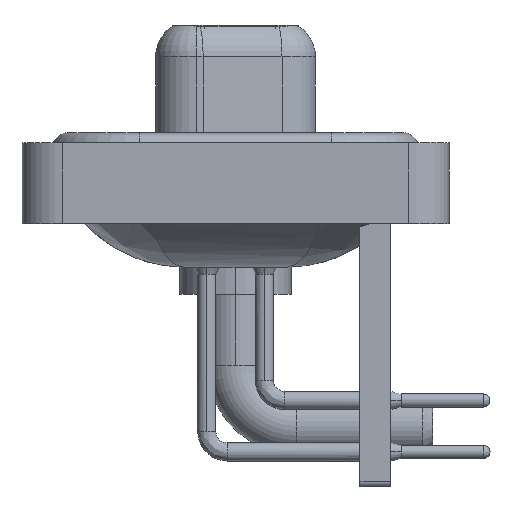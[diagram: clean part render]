
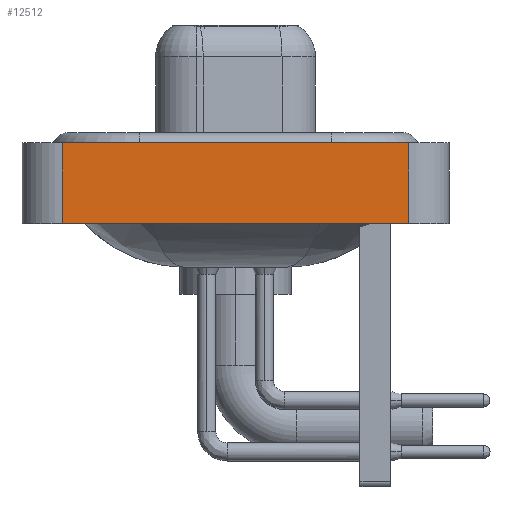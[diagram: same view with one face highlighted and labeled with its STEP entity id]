
A CAD part, left-side view. The second image highlights one B-rep face of the part: STEP entity #12512.
In plain terms, the highlighted planar face has unit normal (-1, 0, 0).
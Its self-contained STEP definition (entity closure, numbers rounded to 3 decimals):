
#1322 = FACE_OUTER_BOUND ( 'NONE', #2373, .T. ) ;
#1960 = DIRECTION ( 'NONE',  ( 0., 0., 1. ) ) ;
#2230 = DIRECTION ( 'NONE',  ( 0., 0., 1. ) ) ;
#2296 = LINE ( 'NONE', #13627, #19000 ) ;
#2373 = EDGE_LOOP ( 'NONE', ( #7023, #11223, #7813, #7846 ) ) ;
#2807 = LINE ( 'NONE', #15602, #14955 ) ;
#3771 = CARTESIAN_POINT ( 'NONE',  ( -7.25, -8.55, -3.6 ) ) ;
#3973 = EDGE_CURVE ( 'NONE', #20625, #4179, #2296, .T. ) ;
#4179 = VERTEX_POINT ( 'NONE', #20316 ) ;
#4591 = AXIS2_PLACEMENT_3D ( 'NONE', #19046, #11079, #2230 ) ;
#4674 = DIRECTION ( 'NONE',  ( 0., -1., 0. ) ) ;
#7023 = ORIENTED_EDGE ( 'NONE', *, *, #14893, .T. ) ;
#7077 = LINE ( 'NONE', #10123, #9894 ) ;
#7105 = DIRECTION ( 'NONE',  ( 0., -1., 0. ) ) ;
#7813 = ORIENTED_EDGE ( 'NONE', *, *, #8123, .F. ) ;
#7846 = ORIENTED_EDGE ( 'NONE', *, *, #8810, .T. ) ;
#8016 = VERTEX_POINT ( 'NONE', #3771 ) ;
#8123 = EDGE_CURVE ( 'NONE', #19703, #20625, #16268, .T. ) ;
#8810 = EDGE_CURVE ( 'NONE', #19703, #8016, #2807, .T. ) ;
#9894 = VECTOR ( 'NONE', #1960, 1000. ) ;
#10123 = CARTESIAN_POINT ( 'NONE',  ( -7.25, -8.55, -3.6 ) ) ;
#10589 = CARTESIAN_POINT ( 'NONE',  ( -7.25, 8.55, 0.4 ) ) ;
#11079 = DIRECTION ( 'NONE',  ( -1., 0., 0. ) ) ;
#11223 = ORIENTED_EDGE ( 'NONE', *, *, #3973, .F. ) ;
#11663 = DIRECTION ( 'NONE',  ( 0., 0., 1. ) ) ;
#11761 = CARTESIAN_POINT ( 'NONE',  ( -7.25, 8.55, -3.6 ) ) ;
#12512 = ADVANCED_FACE ( 'NONE', ( #1322 ), #20617, .T. ) ;
#13627 = CARTESIAN_POINT ( 'NONE',  ( -7.25, -8.55, 0.4 ) ) ;
#14893 = EDGE_CURVE ( 'NONE', #8016, #4179, #7077, .T. ) ;
#14955 = VECTOR ( 'NONE', #4674, 1000. ) ;
#15283 = VECTOR ( 'NONE', #11663, 1000. ) ;
#15602 = CARTESIAN_POINT ( 'NONE',  ( -7.25, -8.55, -3.6 ) ) ;
#16268 = LINE ( 'NONE', #11761, #15283 ) ;
#19000 = VECTOR ( 'NONE', #7105, 1000. ) ;
#19046 = CARTESIAN_POINT ( 'NONE',  ( -7.25, -8.55, -3.6 ) ) ;
#19703 = VERTEX_POINT ( 'NONE', #20304 ) ;
#20304 = CARTESIAN_POINT ( 'NONE',  ( -7.25, 8.55, -3.6 ) ) ;
#20316 = CARTESIAN_POINT ( 'NONE',  ( -7.25, -8.55, 0.4 ) ) ;
#20617 = PLANE ( 'NONE',  #4591 ) ;
#20625 = VERTEX_POINT ( 'NONE', #10589 ) ;
